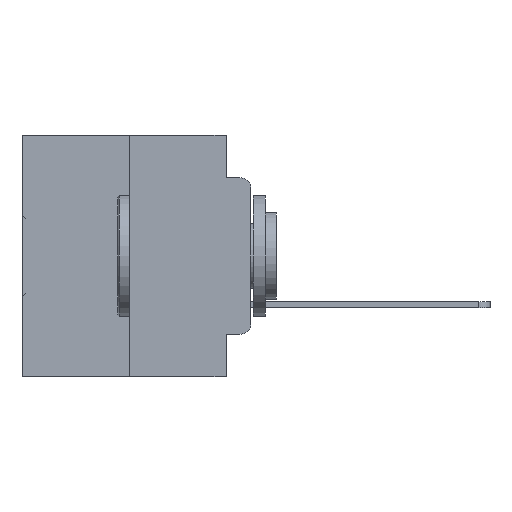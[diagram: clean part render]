
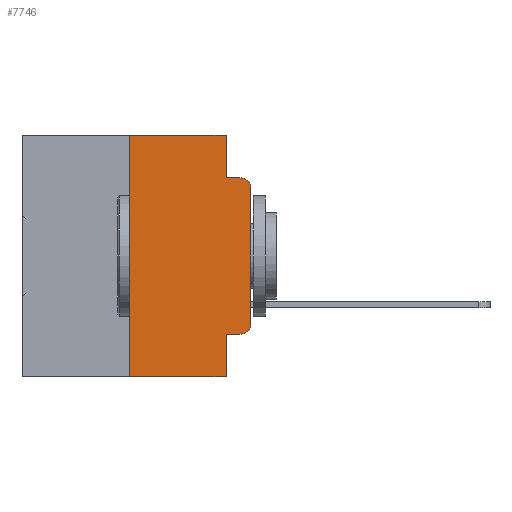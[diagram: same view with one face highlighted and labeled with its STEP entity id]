
A CAD part, left-side view. The second image highlights one B-rep face of the part: STEP entity #7746.
In plain terms, the highlighted planar face has unit normal (-1, 0, 0).
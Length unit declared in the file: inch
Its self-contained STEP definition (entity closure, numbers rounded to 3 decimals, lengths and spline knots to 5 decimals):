
#618 = VERTEX_POINT ( 'NONE', #3378 ) ;
#923 = EDGE_CURVE ( 'NONE', #15112, #1163, #12186, .T. ) ;
#1052 = VECTOR ( 'NONE', #2048, 39.37008 ) ;
#1163 = VERTEX_POINT ( 'NONE', #22699 ) ;
#1744 = CARTESIAN_POINT ( 'NONE',  ( 0., 0.02, -0.1085 ) ) ;
#1883 = EDGE_CURVE ( 'NONE', #29908, #2405, #8063, .T. ) ;
#2048 = DIRECTION ( 'NONE',  ( 0., -1., 0. ) ) ;
#2092 = DIRECTION ( 'NONE',  ( 0., -1., 0. ) ) ;
#2405 = VERTEX_POINT ( 'NONE', #28920 ) ;
#2808 = EDGE_CURVE ( 'NONE', #20031, #1163, #24308, .T. ) ;
#3374 = LINE ( 'NONE', #10597, #30738 ) ;
#3378 = CARTESIAN_POINT ( 'NONE',  ( 0., 0.051, -0.4115 ) ) ;
#3847 = AXIS2_PLACEMENT_3D ( 'NONE', #6531, #25277, #9491 ) ;
#4628 = DIRECTION ( 'NONE',  ( 0., 0., -1. ) ) ;
#4749 = EDGE_CURVE ( 'NONE', #17095, #20031, #3374, .T. ) ;
#5329 = DIRECTION ( 'NONE',  ( 0., -1., 0. ) ) ;
#5379 = LINE ( 'NONE', #13911, #12155 ) ;
#6298 = LINE ( 'NONE', #7726, #7196 ) ;
#6531 = CARTESIAN_POINT ( 'NONE',  ( 0., 0.02, -0.3915 ) ) ;
#7196 = VECTOR ( 'NONE', #28716, 39.37008 ) ;
#7199 = DIRECTION ( 'NONE',  ( 0., -1., 0. ) ) ;
#7726 = CARTESIAN_POINT ( 'NONE',  ( 0., 0.051, 0. ) ) ;
#7746 = ADVANCED_FACE ( 'NONE', ( #10933 ), #13743, .F. ) ;
#8063 = LINE ( 'NONE', #21779, #28183 ) ;
#8163 = DIRECTION ( 'NONE',  ( 0., 0., -1. ) ) ;
#8194 = DIRECTION ( 'NONE',  ( 0., 0., -1. ) ) ;
#9491 = DIRECTION ( 'NONE',  ( 0., 0., -1. ) ) ;
#9711 = ORIENTED_EDGE ( 'NONE', *, *, #4749, .T. ) ;
#10160 = CARTESIAN_POINT ( 'NONE',  ( 0., 0., -0.3915 ) ) ;
#10597 = CARTESIAN_POINT ( 'NONE',  ( 0., 0., 0. ) ) ;
#10640 = AXIS2_PLACEMENT_3D ( 'NONE', #1744, #21171, #4628 ) ;
#10921 = VERTEX_POINT ( 'NONE', #28568 ) ;
#10933 = FACE_OUTER_BOUND ( 'NONE', #30969, .T. ) ;
#11063 = ORIENTED_EDGE ( 'NONE', *, *, #2808, .T. ) ;
#11884 = ORIENTED_EDGE ( 'NONE', *, *, #923, .F. ) ;
#11907 = VERTEX_POINT ( 'NONE', #26158 ) ;
#12155 = VECTOR ( 'NONE', #24210, 39.37008 ) ;
#12186 = LINE ( 'NONE', #21230, #31680 ) ;
#13085 = ORIENTED_EDGE ( 'NONE', *, *, #33359, .F. ) ;
#13511 = CARTESIAN_POINT ( 'NONE',  ( 0., 0.473, -0.5 ) ) ;
#13743 = PLANE ( 'NONE',  #24191 ) ;
#13910 = ORIENTED_EDGE ( 'NONE', *, *, #1883, .F. ) ;
#13911 = CARTESIAN_POINT ( 'NONE',  ( 0., 0.25, 0. ) ) ;
#15112 = VERTEX_POINT ( 'NONE', #33668 ) ;
#16019 = LINE ( 'NONE', #26642, #27773 ) ;
#16196 = LINE ( 'NONE', #23907, #1052 ) ;
#16619 = ORIENTED_EDGE ( 'NONE', *, *, #30218, .F. ) ;
#17095 = VERTEX_POINT ( 'NONE', #10160 ) ;
#17956 = ORIENTED_EDGE ( 'NONE', *, *, #22405, .T. ) ;
#19205 = CARTESIAN_POINT ( 'NONE',  ( 0., 0.473, 0. ) ) ;
#19832 = LINE ( 'NONE', #13511, #25600 ) ;
#20031 = VERTEX_POINT ( 'NONE', #22973 ) ;
#20717 = ORIENTED_EDGE ( 'NONE', *, *, #28543, .F. ) ;
#20782 = CARTESIAN_POINT ( 'NONE',  ( 0., 0.25, 0. ) ) ;
#21171 = DIRECTION ( 'NONE',  ( -1., 0., 0. ) ) ;
#21230 = CARTESIAN_POINT ( 'NONE',  ( 0., 0.051, -0.0885 ) ) ;
#21779 = CARTESIAN_POINT ( 'NONE',  ( 0., 0.473, 0. ) ) ;
#21987 = EDGE_CURVE ( 'NONE', #26238, #17095, #23321, .T. ) ;
#22405 = EDGE_CURVE ( 'NONE', #11907, #10921, #19832, .T. ) ;
#22699 = CARTESIAN_POINT ( 'NONE',  ( 0., 0.02, -0.0885 ) ) ;
#22973 = CARTESIAN_POINT ( 'NONE',  ( 0., 0., -0.1085 ) ) ;
#23321 = CIRCLE ( 'NONE', #3847, 0.02 ) ;
#23427 = ORIENTED_EDGE ( 'NONE', *, *, #26888, .T. ) ;
#23907 = CARTESIAN_POINT ( 'NONE',  ( 0., 0.051, -0.4115 ) ) ;
#24179 = DIRECTION ( 'NONE',  ( 1., 0., 0. ) ) ;
#24191 = AXIS2_PLACEMENT_3D ( 'NONE', #19205, #24179, #8163 ) ;
#24210 = DIRECTION ( 'NONE',  ( 0., 0., 1. ) ) ;
#24245 = ORIENTED_EDGE ( 'NONE', *, *, #21987, .T. ) ;
#24308 = CIRCLE ( 'NONE', #10640, 0.02 ) ;
#25277 = DIRECTION ( 'NONE',  ( -1., 0., 0. ) ) ;
#25600 = VECTOR ( 'NONE', #2092, 39.37008 ) ;
#26158 = CARTESIAN_POINT ( 'NONE',  ( 0., 0.25, -0.5 ) ) ;
#26238 = VERTEX_POINT ( 'NONE', #26601 ) ;
#26601 = CARTESIAN_POINT ( 'NONE',  ( 0., 0.02, -0.4115 ) ) ;
#26642 = CARTESIAN_POINT ( 'NONE',  ( 0., 0.051, 0. ) ) ;
#26888 = EDGE_CURVE ( 'NONE', #618, #26238, #16196, .T. ) ;
#27773 = VECTOR ( 'NONE', #8194, 39.37008 ) ;
#28183 = VECTOR ( 'NONE', #5329, 39.37008 ) ;
#28543 = EDGE_CURVE ( 'NONE', #618, #10921, #6298, .T. ) ;
#28568 = CARTESIAN_POINT ( 'NONE',  ( 0., 0.051, -0.5 ) ) ;
#28716 = DIRECTION ( 'NONE',  ( 0., 0., -1. ) ) ;
#28920 = CARTESIAN_POINT ( 'NONE',  ( 0., 0.051, 0. ) ) ;
#29908 = VERTEX_POINT ( 'NONE', #20782 ) ;
#30218 = EDGE_CURVE ( 'NONE', #11907, #29908, #5379, .T. ) ;
#30738 = VECTOR ( 'NONE', #33471, 39.37008 ) ;
#30969 = EDGE_LOOP ( 'NONE', ( #9711, #11063, #11884, #13085, #13910, #16619, #17956, #20717, #23427, #24245 ) ) ;
#31680 = VECTOR ( 'NONE', #7199, 39.37008 ) ;
#33359 = EDGE_CURVE ( 'NONE', #2405, #15112, #16019, .T. ) ;
#33471 = DIRECTION ( 'NONE',  ( 0., 0., 1. ) ) ;
#33668 = CARTESIAN_POINT ( 'NONE',  ( 0., 0.051, -0.0885 ) ) ;
